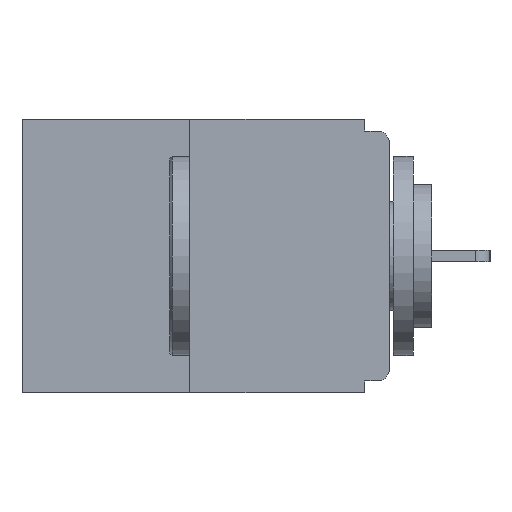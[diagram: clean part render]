
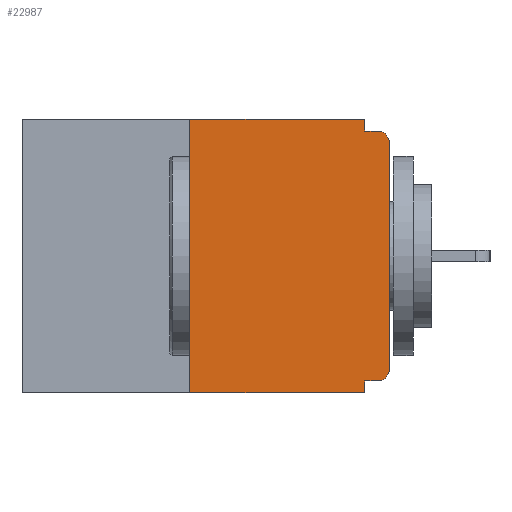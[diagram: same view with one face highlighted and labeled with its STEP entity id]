
A CAD part, left-side view. The second image highlights one B-rep face of the part: STEP entity #22987.
In plain terms, the highlighted planar face has unit normal (-1, 0, 0).
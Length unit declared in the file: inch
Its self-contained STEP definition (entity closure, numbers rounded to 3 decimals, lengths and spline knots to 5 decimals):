
#146 = ORIENTED_EDGE ( 'NONE', *, *, #14728, .F. ) ;
#339 = LINE ( 'NONE', #11600, #4480 ) ;
#506 = CARTESIAN_POINT ( 'NONE',  ( 0., 0., -0.03 ) ) ;
#656 = ORIENTED_EDGE ( 'NONE', *, *, #11537, .F. ) ;
#797 = LINE ( 'NONE', #2701, #10713 ) ;
#1465 = EDGE_LOOP ( 'NONE', ( #18722, #19400, #17267, #656, #146, #13629, #3454, #10500, #15919, #16833 ) ) ;
#1818 = DIRECTION ( 'NONE',  ( 1., 0., 0. ) ) ;
#2070 = DIRECTION ( 'NONE',  ( 0., 0., -1. ) ) ;
#2266 = EDGE_CURVE ( 'NONE', #5413, #3324, #19817, .T. ) ;
#2510 = EDGE_CURVE ( 'NONE', #19411, #8763, #22220, .T. ) ;
#2701 = CARTESIAN_POINT ( 'NONE',  ( 0., 0.46, 0. ) ) ;
#2848 = VERTEX_POINT ( 'NONE', #5051 ) ;
#3106 = LINE ( 'NONE', #19860, #17111 ) ;
#3324 = VERTEX_POINT ( 'NONE', #10438 ) ;
#3454 = ORIENTED_EDGE ( 'NONE', *, *, #16070, .T. ) ;
#4117 = VERTEX_POINT ( 'NONE', #24008 ) ;
#4193 = CARTESIAN_POINT ( 'NONE',  ( 0., 0.015, -0.313 ) ) ;
#4480 = VECTOR ( 'NONE', #13736, 39.37008 ) ;
#4749 = CARTESIAN_POINT ( 'NONE',  ( 0., 0.031, 0. ) ) ;
#4773 = LINE ( 'NONE', #8558, #24661 ) ;
#5051 = CARTESIAN_POINT ( 'NONE',  ( 0., 0.015, -0.328 ) ) ;
#5413 = VERTEX_POINT ( 'NONE', #8626 ) ;
#5838 = FACE_OUTER_BOUND ( 'NONE', #1465, .T. ) ;
#6146 = VERTEX_POINT ( 'NONE', #506 ) ;
#6583 = CARTESIAN_POINT ( 'NONE',  ( 0., 0.031, 0. ) ) ;
#8558 = CARTESIAN_POINT ( 'NONE',  ( 0., 0., -0.015 ) ) ;
#8626 = CARTESIAN_POINT ( 'NONE',  ( 0., 0.25, -0.343 ) ) ;
#8763 = VERTEX_POINT ( 'NONE', #13172 ) ;
#9294 = CIRCLE ( 'NONE', #13741, 0.015 ) ;
#9482 = EDGE_CURVE ( 'NONE', #8763, #19319, #4773, .T. ) ;
#9521 = DIRECTION ( 'NONE',  ( 0., -1., 0. ) ) ;
#9619 = DIRECTION ( 'NONE',  ( -1., 0., 0. ) ) ;
#10438 = CARTESIAN_POINT ( 'NONE',  ( 0., 0.031, -0.343 ) ) ;
#10455 = DIRECTION ( 'NONE',  ( 0., 1., 0. ) ) ;
#10500 = ORIENTED_EDGE ( 'NONE', *, *, #18553, .T. ) ;
#10713 = VECTOR ( 'NONE', #17946, 39.37008 ) ;
#11087 = VERTEX_POINT ( 'NONE', #22426 ) ;
#11537 = EDGE_CURVE ( 'NONE', #11087, #3324, #3106, .T. ) ;
#11600 = CARTESIAN_POINT ( 'NONE',  ( 0., 0.25, 0. ) ) ;
#11979 = VERTEX_POINT ( 'NONE', #18500 ) ;
#12795 = EDGE_CURVE ( 'NONE', #2848, #4117, #19956, .T. ) ;
#13172 = CARTESIAN_POINT ( 'NONE',  ( 0., 0.031, -0.015 ) ) ;
#13475 = VECTOR ( 'NONE', #9521, 39.37008 ) ;
#13582 = CARTESIAN_POINT ( 'NONE',  ( 0., 0.46, -0.343 ) ) ;
#13629 = ORIENTED_EDGE ( 'NONE', *, *, #12795, .T. ) ;
#13736 = DIRECTION ( 'NONE',  ( 0., 0., 1. ) ) ;
#13741 = AXIS2_PLACEMENT_3D ( 'NONE', #14191, #17701, #17586 ) ;
#13839 = LINE ( 'NONE', #16086, #17329 ) ;
#13858 = EDGE_CURVE ( 'NONE', #11979, #19411, #797, .T. ) ;
#14191 = CARTESIAN_POINT ( 'NONE',  ( 0., 0.015, -0.03 ) ) ;
#14670 = DIRECTION ( 'NONE',  ( 0., 0., -1. ) ) ;
#14728 = EDGE_CURVE ( 'NONE', #2848, #11087, #16132, .T. ) ;
#15302 = CARTESIAN_POINT ( 'NONE',  ( 0., 0.46, 0. ) ) ;
#15919 = ORIENTED_EDGE ( 'NONE', *, *, #9482, .F. ) ;
#16070 = EDGE_CURVE ( 'NONE', #4117, #6146, #13839, .T. ) ;
#16086 = CARTESIAN_POINT ( 'NONE',  ( 0., 0., 0. ) ) ;
#16132 = LINE ( 'NONE', #21424, #17571 ) ;
#16833 = ORIENTED_EDGE ( 'NONE', *, *, #2510, .F. ) ;
#17111 = VECTOR ( 'NONE', #19983, 39.37008 ) ;
#17198 = DIRECTION ( 'NONE',  ( 0., 0., -1. ) ) ;
#17267 = ORIENTED_EDGE ( 'NONE', *, *, #2266, .T. ) ;
#17329 = VECTOR ( 'NONE', #23760, 39.37008 ) ;
#17571 = VECTOR ( 'NONE', #10455, 39.37008 ) ;
#17586 = DIRECTION ( 'NONE',  ( 0., 0., -1. ) ) ;
#17701 = DIRECTION ( 'NONE',  ( -1., 0., 0. ) ) ;
#17864 = CARTESIAN_POINT ( 'NONE',  ( 0., 0.015, -0.015 ) ) ;
#17946 = DIRECTION ( 'NONE',  ( 0., -1., 0. ) ) ;
#18397 = DIRECTION ( 'NONE',  ( 0., -1., 0. ) ) ;
#18500 = CARTESIAN_POINT ( 'NONE',  ( 0., 0.25, 0. ) ) ;
#18553 = EDGE_CURVE ( 'NONE', #6146, #19319, #9294, .T. ) ;
#18722 = ORIENTED_EDGE ( 'NONE', *, *, #13858, .F. ) ;
#19075 = PLANE ( 'NONE',  #21828 ) ;
#19319 = VERTEX_POINT ( 'NONE', #17864 ) ;
#19400 = ORIENTED_EDGE ( 'NONE', *, *, #22109, .F. ) ;
#19411 = VERTEX_POINT ( 'NONE', #4749 ) ;
#19817 = LINE ( 'NONE', #13582, #13475 ) ;
#19860 = CARTESIAN_POINT ( 'NONE',  ( 0., 0.031, -0.343 ) ) ;
#19956 = CIRCLE ( 'NONE', #24808, 0.015 ) ;
#19983 = DIRECTION ( 'NONE',  ( 0., 0., -1. ) ) ;
#21424 = CARTESIAN_POINT ( 'NONE',  ( 0., 0., -0.328 ) ) ;
#21828 = AXIS2_PLACEMENT_3D ( 'NONE', #15302, #1818, #17198 ) ;
#22109 = EDGE_CURVE ( 'NONE', #5413, #11979, #339, .T. ) ;
#22220 = LINE ( 'NONE', #6583, #24326 ) ;
#22426 = CARTESIAN_POINT ( 'NONE',  ( 0., 0.031, -0.328 ) ) ;
#22987 = ADVANCED_FACE ( 'NONE', ( #5838 ), #19075, .F. ) ;
#23760 = DIRECTION ( 'NONE',  ( 0., 0., 1. ) ) ;
#24008 = CARTESIAN_POINT ( 'NONE',  ( 0., 0., -0.313 ) ) ;
#24326 = VECTOR ( 'NONE', #14670, 39.37008 ) ;
#24661 = VECTOR ( 'NONE', #18397, 39.37008 ) ;
#24808 = AXIS2_PLACEMENT_3D ( 'NONE', #4193, #9619, #2070 ) ;
